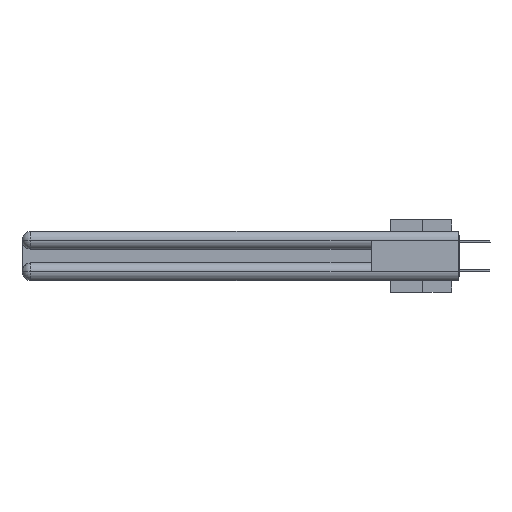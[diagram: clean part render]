
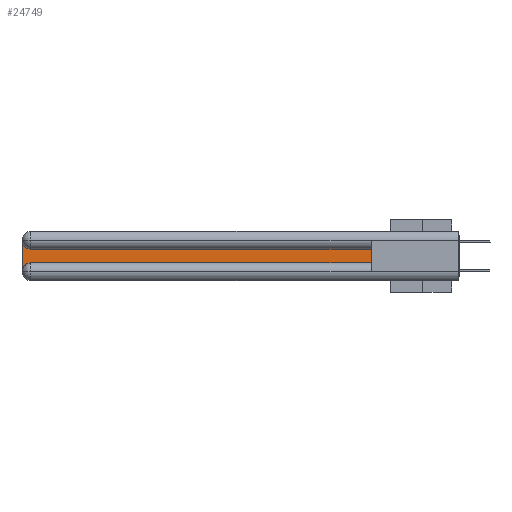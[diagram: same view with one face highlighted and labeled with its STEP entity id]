
A CAD part, left-side view. The second image highlights one B-rep face of the part: STEP entity #24749.
In plain terms, the highlighted planar face has unit normal (-1, 0, 0).
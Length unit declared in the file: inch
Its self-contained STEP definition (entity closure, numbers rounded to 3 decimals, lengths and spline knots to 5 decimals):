
#399 = CARTESIAN_POINT ( 'NONE',  ( 0.075, 3., -0.1225 ) ) ;
#461 = CARTESIAN_POINT ( 'NONE',  ( 0.075, 3., -0.2175 ) ) ;
#1177 = VERTEX_POINT ( 'NONE', #16290 ) ;
#1193 = ORIENTED_EDGE ( 'NONE', *, *, #19375, .T. ) ;
#1414 = DIRECTION ( 'NONE',  ( 1., 0., 0. ) ) ;
#1518 = CARTESIAN_POINT ( 'NONE',  ( 0.075, 3., -0.0625 ) ) ;
#2955 = PLANE ( 'NONE',  #14122 ) ;
#3306 = LINE ( 'NONE', #5769, #20383 ) ;
#3505 = DIRECTION ( 'NONE',  ( 0., 0., 1. ) ) ;
#3613 = AXIS2_PLACEMENT_3D ( 'NONE', #5467, #27527, #17961 ) ;
#3746 = DIRECTION ( 'NONE',  ( 0., 0., -1. ) ) ;
#4118 = DIRECTION ( 'NONE',  ( 0., -1., 0. ) ) ;
#5467 = CARTESIAN_POINT ( 'NONE',  ( 0.075, 2.94, -0.0625 ) ) ;
#5769 = CARTESIAN_POINT ( 'NONE',  ( 0.075, 0.6, -0.2175 ) ) ;
#5779 = VECTOR ( 'NONE', #10041, 39.37008 ) ;
#6425 = CIRCLE ( 'NONE', #3613, 0.06 ) ;
#6492 = LINE ( 'NONE', #461, #5779 ) ;
#7890 = CARTESIAN_POINT ( 'NONE',  ( 0.075, 0.6, -0.1225 ) ) ;
#8449 = ORIENTED_EDGE ( 'NONE', *, *, #10468, .T. ) ;
#8749 = EDGE_CURVE ( 'NONE', #10163, #13208, #6425, .T. ) ;
#9058 = CARTESIAN_POINT ( 'NONE',  ( 0.075, 2.94, -0.2175 ) ) ;
#9883 = CARTESIAN_POINT ( 'NONE',  ( 0.075, 2.94, -0.1225 ) ) ;
#10041 = DIRECTION ( 'NONE',  ( 0., 0., -1. ) ) ;
#10163 = VERTEX_POINT ( 'NONE', #9883 ) ;
#10468 = EDGE_CURVE ( 'NONE', #1177, #10163, #22669, .T. ) ;
#12157 = DIRECTION ( 'NONE',  ( 0., 1., 0. ) ) ;
#13208 = VERTEX_POINT ( 'NONE', #1518 ) ;
#13285 = EDGE_LOOP ( 'NONE', ( #8449, #16926, #1193, #21303, #25595, #23629 ) ) ;
#14122 = AXIS2_PLACEMENT_3D ( 'NONE', #399, #23747, #28581 ) ;
#14315 = FACE_OUTER_BOUND ( 'NONE', #13285, .T. ) ;
#15438 = CIRCLE ( 'NONE', #24567, 0.06 ) ;
#15525 = VERTEX_POINT ( 'NONE', #26980 ) ;
#15659 = VECTOR ( 'NONE', #3505, 39.37008 ) ;
#16290 = CARTESIAN_POINT ( 'NONE',  ( 0.075, 0.6, -0.1225 ) ) ;
#16515 = VECTOR ( 'NONE', #12157, 39.37008 ) ;
#16926 = ORIENTED_EDGE ( 'NONE', *, *, #8749, .T. ) ;
#17444 = CARTESIAN_POINT ( 'NONE',  ( 0.075, 0.6, -0.2175 ) ) ;
#17700 = CARTESIAN_POINT ( 'NONE',  ( 0.075, 2.94, -0.2775 ) ) ;
#17789 = EDGE_CURVE ( 'NONE', #28885, #29030, #3306, .T. ) ;
#17961 = DIRECTION ( 'NONE',  ( 0., 0., -1. ) ) ;
#18264 = EDGE_CURVE ( 'NONE', #29030, #1177, #27914, .T. ) ;
#19375 = EDGE_CURVE ( 'NONE', #13208, #15525, #6492, .T. ) ;
#20383 = VECTOR ( 'NONE', #4118, 39.37008 ) ;
#21303 = ORIENTED_EDGE ( 'NONE', *, *, #21798, .T. ) ;
#21798 = EDGE_CURVE ( 'NONE', #15525, #28885, #15438, .T. ) ;
#22669 = LINE ( 'NONE', #7890, #16515 ) ;
#23629 = ORIENTED_EDGE ( 'NONE', *, *, #18264, .T. ) ;
#23747 = DIRECTION ( 'NONE',  ( 1., 0., 0. ) ) ;
#24567 = AXIS2_PLACEMENT_3D ( 'NONE', #17700, #1414, #3746 ) ;
#24749 = ADVANCED_FACE ( 'NONE', ( #14315 ), #2955, .F. ) ;
#25595 = ORIENTED_EDGE ( 'NONE', *, *, #17789, .T. ) ;
#26980 = CARTESIAN_POINT ( 'NONE',  ( 0.075, 3., -0.2775 ) ) ;
#27527 = DIRECTION ( 'NONE',  ( 1., 0., 0. ) ) ;
#27914 = LINE ( 'NONE', #17444, #15659 ) ;
#27947 = CARTESIAN_POINT ( 'NONE',  ( 0.075, 0.6, -0.2175 ) ) ;
#28581 = DIRECTION ( 'NONE',  ( 0., 0., -1. ) ) ;
#28885 = VERTEX_POINT ( 'NONE', #9058 ) ;
#29030 = VERTEX_POINT ( 'NONE', #27947 ) ;
